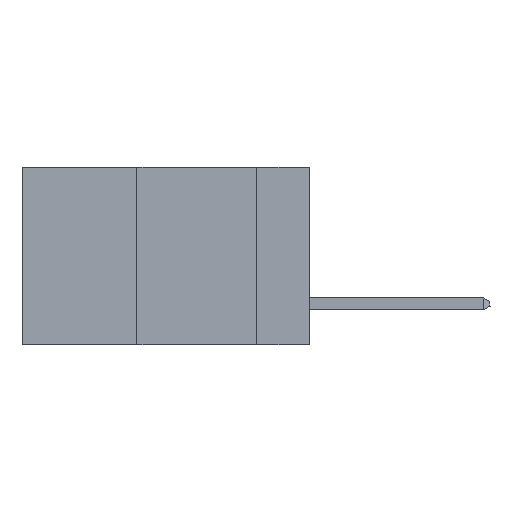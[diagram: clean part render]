
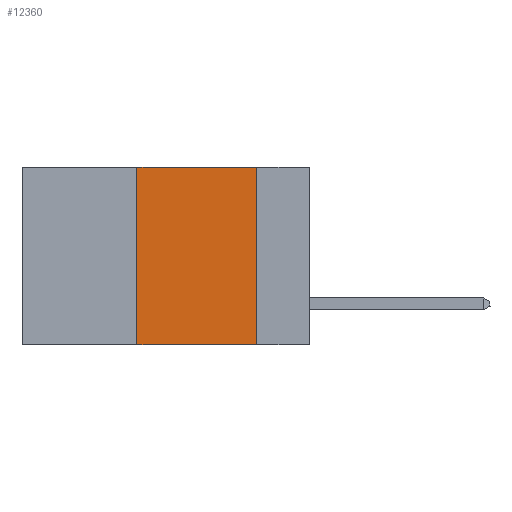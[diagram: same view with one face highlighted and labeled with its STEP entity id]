
A CAD part, left-side view. The second image highlights one B-rep face of the part: STEP entity #12360.
In plain terms, the highlighted planar face has unit normal (-1, 0, 0).
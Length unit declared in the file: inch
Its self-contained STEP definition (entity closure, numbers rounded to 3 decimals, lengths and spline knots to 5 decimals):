
#46 = EDGE_CURVE ( 'NONE', #2274, #3571, #15097, .T. ) ;
#728 = VECTOR ( 'NONE', #7878, 39.37008 ) ;
#733 = DIRECTION ( 'NONE',  ( 1., 0., 0. ) ) ;
#1158 = CARTESIAN_POINT ( 'NONE',  ( 0., 0.6, -0.37 ) ) ;
#1552 = CARTESIAN_POINT ( 'NONE',  ( 0., 0.6, 0. ) ) ;
#1763 = AXIS2_PLACEMENT_3D ( 'NONE', #2170, #733, #9233 ) ;
#2152 = FACE_OUTER_BOUND ( 'NONE', #7145, .T. ) ;
#2170 = CARTESIAN_POINT ( 'NONE',  ( 0., 0.6, 0. ) ) ;
#2274 = VERTEX_POINT ( 'NONE', #4067 ) ;
#2895 = VECTOR ( 'NONE', #8080, 39.37008 ) ;
#3316 = ORIENTED_EDGE ( 'NONE', *, *, #3481, .F. ) ;
#3481 = EDGE_CURVE ( 'NONE', #2274, #7372, #15112, .T. ) ;
#3571 = VERTEX_POINT ( 'NONE', #8572 ) ;
#4067 = CARTESIAN_POINT ( 'NONE',  ( 0., 0.36, -0.37 ) ) ;
#4954 = VECTOR ( 'NONE', #9583, 39.37008 ) ;
#6179 = EDGE_CURVE ( 'NONE', #7372, #8802, #11831, .T. ) ;
#6844 = VECTOR ( 'NONE', #12033, 39.37008 ) ;
#6903 = PLANE ( 'NONE',  #1763 ) ;
#7145 = EDGE_LOOP ( 'NONE', ( #13875, #11483, #3316, #12621 ) ) ;
#7372 = VERTEX_POINT ( 'NONE', #13678 ) ;
#7708 = CARTESIAN_POINT ( 'NONE',  ( 0., 0.36, 0. ) ) ;
#7878 = DIRECTION ( 'NONE',  ( 0., -1., 0. ) ) ;
#8080 = DIRECTION ( 'NONE',  ( 0., 0., 1. ) ) ;
#8379 = LINE ( 'NONE', #10685, #6844 ) ;
#8572 = CARTESIAN_POINT ( 'NONE',  ( 0., 0.11, -0.37 ) ) ;
#8802 = VERTEX_POINT ( 'NONE', #14153 ) ;
#9233 = DIRECTION ( 'NONE',  ( 0., 0., -1. ) ) ;
#9583 = DIRECTION ( 'NONE',  ( 0., -1., 0. ) ) ;
#10685 = CARTESIAN_POINT ( 'NONE',  ( 0., 0.11, 0. ) ) ;
#11483 = ORIENTED_EDGE ( 'NONE', *, *, #6179, .F. ) ;
#11831 = LINE ( 'NONE', #1552, #728 ) ;
#12033 = DIRECTION ( 'NONE',  ( 0., 0., -1. ) ) ;
#12360 = ADVANCED_FACE ( 'NONE', ( #2152 ), #6903, .F. ) ;
#12581 = EDGE_CURVE ( 'NONE', #8802, #3571, #8379, .T. ) ;
#12621 = ORIENTED_EDGE ( 'NONE', *, *, #46, .T. ) ;
#13678 = CARTESIAN_POINT ( 'NONE',  ( 0., 0.36, 0. ) ) ;
#13875 = ORIENTED_EDGE ( 'NONE', *, *, #12581, .F. ) ;
#14153 = CARTESIAN_POINT ( 'NONE',  ( 0., 0.11, 0. ) ) ;
#15097 = LINE ( 'NONE', #1158, #4954 ) ;
#15112 = LINE ( 'NONE', #7708, #2895 ) ;
